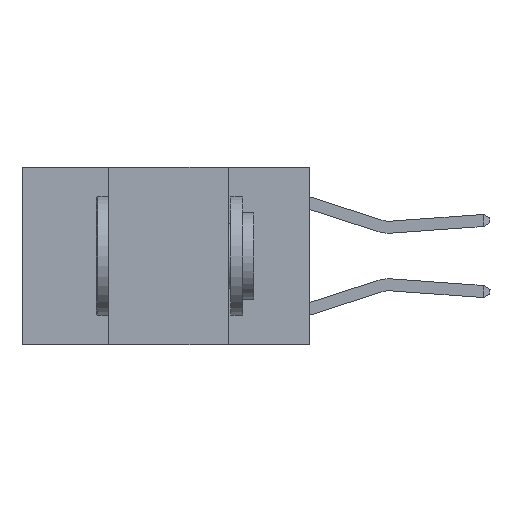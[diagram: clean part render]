
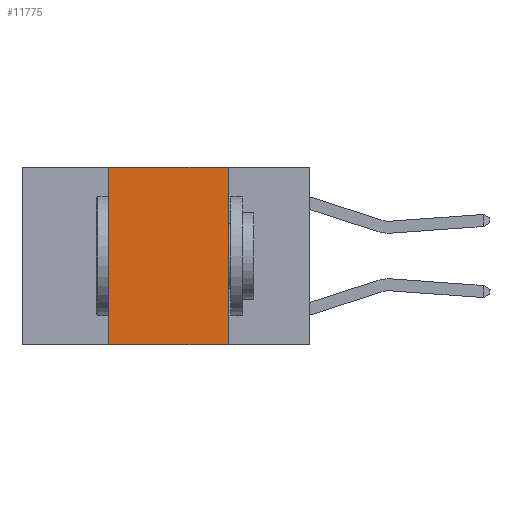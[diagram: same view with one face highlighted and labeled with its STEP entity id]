
A CAD part, left-side view. The second image highlights one B-rep face of the part: STEP entity #11775.
In plain terms, the highlighted planar face has unit normal (-1, 0, 0).
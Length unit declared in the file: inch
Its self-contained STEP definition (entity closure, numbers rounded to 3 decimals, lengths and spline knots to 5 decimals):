
#246 = ORIENTED_EDGE ( 'NONE', *, *, #13263, .T. ) ;
#773 = AXIS2_PLACEMENT_3D ( 'NONE', #14747, #17817, #17908 ) ;
#1788 = LINE ( 'NONE', #9909, #2846 ) ;
#1828 = LINE ( 'NONE', #14748, #3205 ) ;
#2554 = EDGE_LOOP ( 'NONE', ( #17588, #12638, #17469, #246 ) ) ;
#2846 = VECTOR ( 'NONE', #18350, 39.37008 ) ;
#3205 = VECTOR ( 'NONE', #11701, 39.37008 ) ;
#4847 = VERTEX_POINT ( 'NONE', #16481 ) ;
#4870 = VERTEX_POINT ( 'NONE', #15869 ) ;
#6521 = VERTEX_POINT ( 'NONE', #11281 ) ;
#6717 = DIRECTION ( 'NONE',  ( 0., -1., 0. ) ) ;
#7302 = CARTESIAN_POINT ( 'NONE',  ( 0., 0.42, -0.37 ) ) ;
#8022 = LINE ( 'NONE', #15336, #17006 ) ;
#8506 = EDGE_CURVE ( 'NONE', #14234, #6521, #15125, .T. ) ;
#9909 = CARTESIAN_POINT ( 'NONE',  ( 0., 0.17, 0. ) ) ;
#11281 = CARTESIAN_POINT ( 'NONE',  ( 0., 0.42, 0. ) ) ;
#11555 = VECTOR ( 'NONE', #13543, 39.37008 ) ;
#11701 = DIRECTION ( 'NONE',  ( 0., -1., 0. ) ) ;
#11775 = ADVANCED_FACE ( 'NONE', ( #15114 ), #15006, .F. ) ;
#12542 = EDGE_CURVE ( 'NONE', #4870, #4847, #1788, .T. ) ;
#12638 = ORIENTED_EDGE ( 'NONE', *, *, #15273, .F. ) ;
#13263 = EDGE_CURVE ( 'NONE', #14234, #4847, #8022, .T. ) ;
#13543 = DIRECTION ( 'NONE',  ( 0., 0., 1. ) ) ;
#14234 = VERTEX_POINT ( 'NONE', #7302 ) ;
#14747 = CARTESIAN_POINT ( 'NONE',  ( 0., 0.6, 0. ) ) ;
#14748 = CARTESIAN_POINT ( 'NONE',  ( 0., 0.6, 0. ) ) ;
#15006 = PLANE ( 'NONE',  #773 ) ;
#15114 = FACE_OUTER_BOUND ( 'NONE', #2554, .T. ) ;
#15125 = LINE ( 'NONE', #16354, #11555 ) ;
#15273 = EDGE_CURVE ( 'NONE', #6521, #4870, #1828, .T. ) ;
#15336 = CARTESIAN_POINT ( 'NONE',  ( 0., 0.6, -0.37 ) ) ;
#15869 = CARTESIAN_POINT ( 'NONE',  ( 0., 0.17, 0. ) ) ;
#16354 = CARTESIAN_POINT ( 'NONE',  ( 0., 0.42, 0. ) ) ;
#16481 = CARTESIAN_POINT ( 'NONE',  ( 0., 0.17, -0.37 ) ) ;
#17006 = VECTOR ( 'NONE', #6717, 39.37008 ) ;
#17469 = ORIENTED_EDGE ( 'NONE', *, *, #8506, .F. ) ;
#17588 = ORIENTED_EDGE ( 'NONE', *, *, #12542, .F. ) ;
#17817 = DIRECTION ( 'NONE',  ( 1., 0., 0. ) ) ;
#17908 = DIRECTION ( 'NONE',  ( 0., 0., -1. ) ) ;
#18350 = DIRECTION ( 'NONE',  ( 0., 0., -1. ) ) ;
